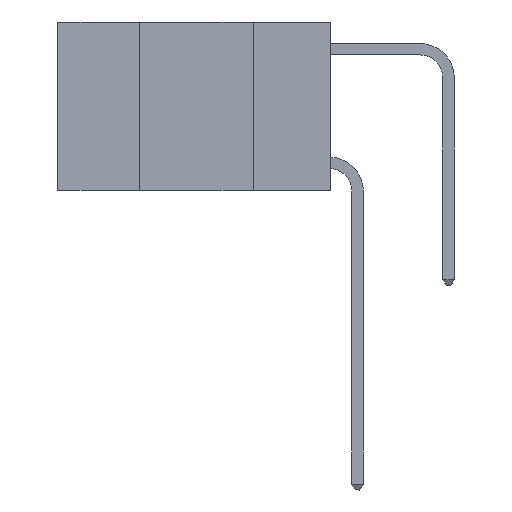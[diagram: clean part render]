
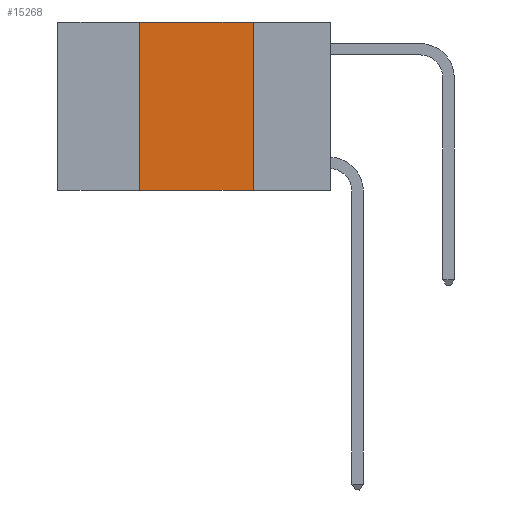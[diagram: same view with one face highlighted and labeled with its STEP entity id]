
A CAD part, left-side view. The second image highlights one B-rep face of the part: STEP entity #15268.
In plain terms, the highlighted planar face has unit normal (-1, 0, 0).
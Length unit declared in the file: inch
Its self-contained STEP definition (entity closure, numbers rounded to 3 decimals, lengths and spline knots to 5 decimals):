
#150 = CARTESIAN_POINT ( 'NONE',  ( 0., 0.17, 0. ) ) ;
#860 = EDGE_CURVE ( 'NONE', #1294, #1189, #18074, .T. ) ;
#1189 = VERTEX_POINT ( 'NONE', #4169 ) ;
#1294 = VERTEX_POINT ( 'NONE', #15049 ) ;
#1409 = ORIENTED_EDGE ( 'NONE', *, *, #10020, .F. ) ;
#1839 = DIRECTION ( 'NONE',  ( 0., 0., -1. ) ) ;
#2013 = EDGE_CURVE ( 'NONE', #1294, #5855, #19250, .T. ) ;
#2233 = EDGE_CURVE ( 'NONE', #5559, #5855, #14836, .T. ) ;
#2645 = FACE_OUTER_BOUND ( 'NONE', #18631, .T. ) ;
#2923 = CARTESIAN_POINT ( 'NONE',  ( 0., 0.6, 0. ) ) ;
#3410 = AXIS2_PLACEMENT_3D ( 'NONE', #2923, #9638, #18065 ) ;
#3841 = ORIENTED_EDGE ( 'NONE', *, *, #2013, .T. ) ;
#4169 = CARTESIAN_POINT ( 'NONE',  ( 0., 0.42, 0. ) ) ;
#4703 = CARTESIAN_POINT ( 'NONE',  ( 0., 0.17, 0. ) ) ;
#5219 = VECTOR ( 'NONE', #20573, 39.37008 ) ;
#5559 = VERTEX_POINT ( 'NONE', #4703 ) ;
#5855 = VERTEX_POINT ( 'NONE', #9284 ) ;
#9113 = LINE ( 'NONE', #17224, #5219 ) ;
#9284 = CARTESIAN_POINT ( 'NONE',  ( 0., 0.17, -0.37 ) ) ;
#9638 = DIRECTION ( 'NONE',  ( 1., 0., 0. ) ) ;
#10020 = EDGE_CURVE ( 'NONE', #1189, #5559, #9113, .T. ) ;
#13123 = CARTESIAN_POINT ( 'NONE',  ( 0., 0.6, -0.37 ) ) ;
#13513 = ORIENTED_EDGE ( 'NONE', *, *, #860, .F. ) ;
#13629 = VECTOR ( 'NONE', #21323, 39.37008 ) ;
#14309 = VECTOR ( 'NONE', #1839, 39.37008 ) ;
#14781 = DIRECTION ( 'NONE',  ( 0., -1., 0. ) ) ;
#14813 = VECTOR ( 'NONE', #14781, 39.37008 ) ;
#14836 = LINE ( 'NONE', #150, #14309 ) ;
#15049 = CARTESIAN_POINT ( 'NONE',  ( 0., 0.42, -0.37 ) ) ;
#15268 = ADVANCED_FACE ( 'NONE', ( #2645 ), #19583, .F. ) ;
#17224 = CARTESIAN_POINT ( 'NONE',  ( 0., 0.6, 0. ) ) ;
#18065 = DIRECTION ( 'NONE',  ( 0., 0., -1. ) ) ;
#18074 = LINE ( 'NONE', #18206, #13629 ) ;
#18206 = CARTESIAN_POINT ( 'NONE',  ( 0., 0.42, 0. ) ) ;
#18631 = EDGE_LOOP ( 'NONE', ( #20465, #1409, #13513, #3841 ) ) ;
#19250 = LINE ( 'NONE', #13123, #14813 ) ;
#19583 = PLANE ( 'NONE',  #3410 ) ;
#20465 = ORIENTED_EDGE ( 'NONE', *, *, #2233, .F. ) ;
#20573 = DIRECTION ( 'NONE',  ( 0., -1., 0. ) ) ;
#21323 = DIRECTION ( 'NONE',  ( 0., 0., 1. ) ) ;
